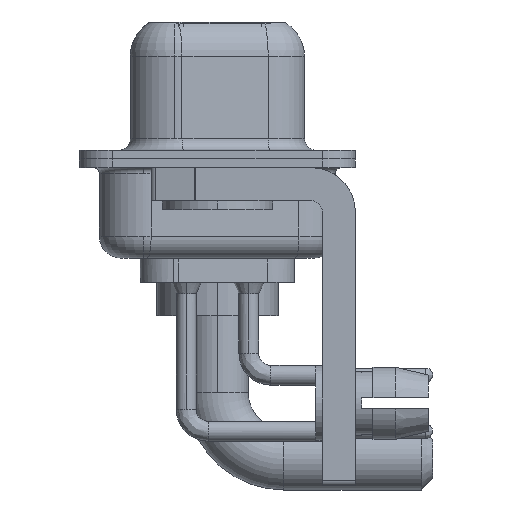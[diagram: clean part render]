
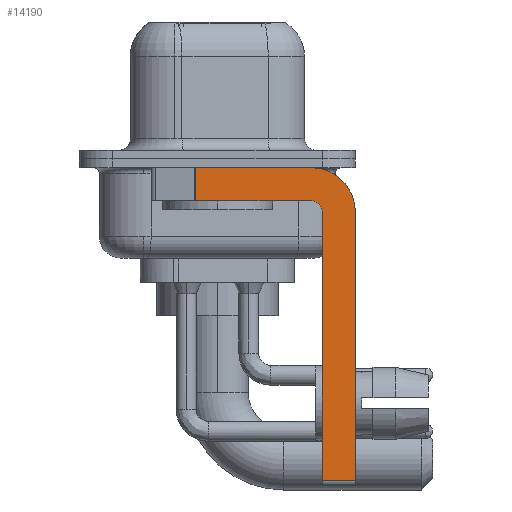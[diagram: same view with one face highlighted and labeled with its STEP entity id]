
A CAD part, left-side view. The second image highlights one B-rep face of the part: STEP entity #14190.
In plain terms, the highlighted planar face has unit normal (-1, 0, 0).
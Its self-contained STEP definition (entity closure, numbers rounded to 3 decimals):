
#28 = DIRECTION ( 'NONE',  ( 0., 0., 1. ) ) ;
#148 = ORIENTED_EDGE ( 'NONE', *, *, #9428, .F. ) ;
#519 = CARTESIAN_POINT ( 'NONE',  ( -2.9, 3., -0.4 ) ) ;
#1032 = EDGE_CURVE ( 'NONE', #3648, #14366, #2872, .T. ) ;
#1651 = AXIS2_PLACEMENT_3D ( 'NONE', #8030, #17241, #28 ) ;
#1808 = VECTOR ( 'NONE', #12838, 1000. ) ;
#2106 = FACE_OUTER_BOUND ( 'NONE', #9047, .T. ) ;
#2872 = LINE ( 'NONE', #16039, #20661 ) ;
#3057 = LINE ( 'NONE', #519, #16281 ) ;
#3648 = VERTEX_POINT ( 'NONE', #11874 ) ;
#4095 = VECTOR ( 'NONE', #14989, 1000. ) ;
#4515 = CARTESIAN_POINT ( 'NONE',  ( -2.9, 0.978, -1.9 ) ) ;
#5378 = AXIS2_PLACEMENT_3D ( 'NONE', #6291, #15639, #23372 ) ;
#5912 = CARTESIAN_POINT ( 'NONE',  ( -2.9, -4.25, -2.4 ) ) ;
#6260 = CARTESIAN_POINT ( 'NONE',  ( -2.9, -4.25, -1.9 ) ) ;
#6291 = CARTESIAN_POINT ( 'NONE',  ( -2.9, -4.25, -2.4 ) ) ;
#6778 = CARTESIAN_POINT ( 'NONE',  ( -2.9, -4.25, -0.4 ) ) ;
#7530 = LINE ( 'NONE', #15229, #1808 ) ;
#7951 = DIRECTION ( 'NONE',  ( 0., 0., -1. ) ) ;
#8030 = CARTESIAN_POINT ( 'NONE',  ( -2.9, -4.25, -2.4 ) ) ;
#8269 = DIRECTION ( 'NONE',  ( 0., -1., 0. ) ) ;
#8669 = ORIENTED_EDGE ( 'NONE', *, *, #1032, .F. ) ;
#8712 = DIRECTION ( 'NONE',  ( 0., 0., 1. ) ) ;
#9047 = EDGE_LOOP ( 'NONE', ( #18289, #14085, #19158, #148, #8669, #9290, #13415, #15300 ) ) ;
#9290 = ORIENTED_EDGE ( 'NONE', *, *, #23810, .T. ) ;
#9428 = EDGE_CURVE ( 'NONE', #14366, #19163, #12575, .T. ) ;
#9834 = VERTEX_POINT ( 'NONE', #15799 ) ;
#10206 = DIRECTION ( 'NONE',  ( 0., 0., -1. ) ) ;
#11256 = VERTEX_POINT ( 'NONE', #6778 ) ;
#11536 = EDGE_CURVE ( 'NONE', #19163, #23615, #24514, .T. ) ;
#11556 = VECTOR ( 'NONE', #7951, 1000. ) ;
#11874 = CARTESIAN_POINT ( 'NONE',  ( -2.9, -4.75, -14.55 ) ) ;
#12237 = PLANE ( 'NONE',  #12632 ) ;
#12575 = CIRCLE ( 'NONE', #1651, 0.5 ) ;
#12632 = AXIS2_PLACEMENT_3D ( 'NONE', #5912, #19691, #10206 ) ;
#12838 = DIRECTION ( 'NONE',  ( 0., -1., 0. ) ) ;
#13415 = ORIENTED_EDGE ( 'NONE', *, *, #24678, .F. ) ;
#13880 = CIRCLE ( 'NONE', #5378, 2. ) ;
#14085 = ORIENTED_EDGE ( 'NONE', *, *, #15207, .T. ) ;
#14190 = ADVANCED_FACE ( 'NONE', ( #2106 ), #12237, .F. ) ;
#14366 = VERTEX_POINT ( 'NONE', #21985 ) ;
#14466 = EDGE_CURVE ( 'NONE', #17753, #11256, #3057, .T. ) ;
#14989 = DIRECTION ( 'NONE',  ( 0., 1., 0. ) ) ;
#15207 = EDGE_CURVE ( 'NONE', #17753, #23615, #23224, .T. ) ;
#15229 = CARTESIAN_POINT ( 'NONE',  ( -2.9, -4.25, -14.55 ) ) ;
#15300 = ORIENTED_EDGE ( 'NONE', *, *, #22146, .F. ) ;
#15639 = DIRECTION ( 'NONE',  ( 1., 0., 0. ) ) ;
#15683 = CARTESIAN_POINT ( 'NONE',  ( -2.9, -6.25, -14.55 ) ) ;
#15799 = CARTESIAN_POINT ( 'NONE',  ( -2.9, -6.25, -2.4 ) ) ;
#16039 = CARTESIAN_POINT ( 'NONE',  ( -2.9, -4.75, -14.8 ) ) ;
#16105 = VERTEX_POINT ( 'NONE', #15683 ) ;
#16281 = VECTOR ( 'NONE', #8269, 1000. ) ;
#17241 = DIRECTION ( 'NONE',  ( -1., 0., 0. ) ) ;
#17753 = VERTEX_POINT ( 'NONE', #24982 ) ;
#17884 = CARTESIAN_POINT ( 'NONE',  ( -2.9, 0.978, -1.9 ) ) ;
#18289 = ORIENTED_EDGE ( 'NONE', *, *, #14466, .F. ) ;
#19120 = VECTOR ( 'NONE', #23478, 1000. ) ;
#19158 = ORIENTED_EDGE ( 'NONE', *, *, #11536, .F. ) ;
#19163 = VERTEX_POINT ( 'NONE', #6260 ) ;
#19691 = DIRECTION ( 'NONE',  ( 1., 0., 0. ) ) ;
#20567 = CARTESIAN_POINT ( 'NONE',  ( -2.9, -4.25, -1.9 ) ) ;
#20661 = VECTOR ( 'NONE', #8712, 1000. ) ;
#21612 = CARTESIAN_POINT ( 'NONE',  ( -2.9, -6.25, -2.4 ) ) ;
#21985 = CARTESIAN_POINT ( 'NONE',  ( -2.9, -4.75, -2.4 ) ) ;
#22146 = EDGE_CURVE ( 'NONE', #11256, #9834, #13880, .T. ) ;
#23224 = LINE ( 'NONE', #17884, #19120 ) ;
#23372 = DIRECTION ( 'NONE',  ( 0., 0., -1. ) ) ;
#23379 = LINE ( 'NONE', #21612, #11556 ) ;
#23478 = DIRECTION ( 'NONE',  ( 0., 0., -1. ) ) ;
#23615 = VERTEX_POINT ( 'NONE', #4515 ) ;
#23810 = EDGE_CURVE ( 'NONE', #3648, #16105, #7530, .T. ) ;
#24514 = LINE ( 'NONE', #20567, #4095 ) ;
#24678 = EDGE_CURVE ( 'NONE', #9834, #16105, #23379, .T. ) ;
#24982 = CARTESIAN_POINT ( 'NONE',  ( -2.9, 0.978, -0.4 ) ) ;
